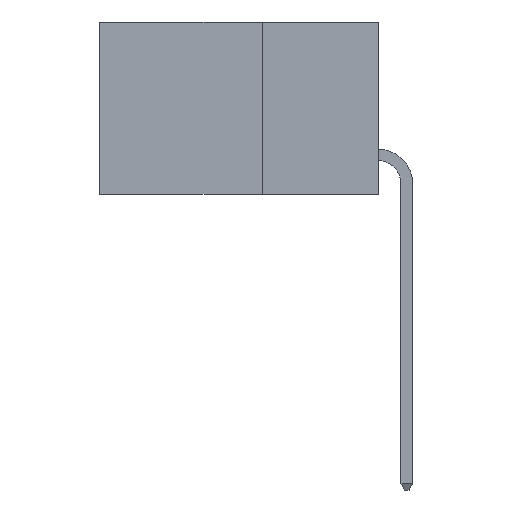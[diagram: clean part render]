
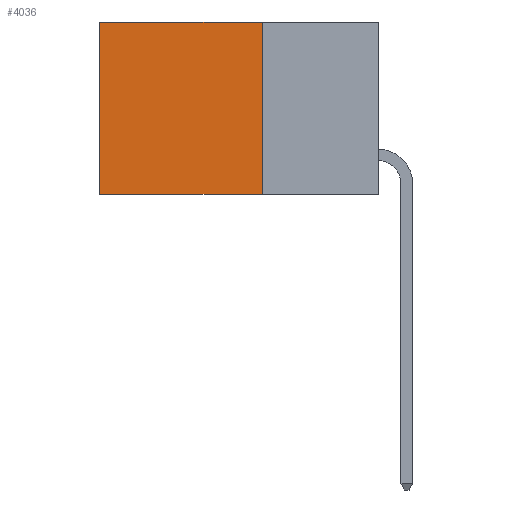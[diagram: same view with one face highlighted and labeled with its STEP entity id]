
A CAD part, left-side view. The second image highlights one B-rep face of the part: STEP entity #4036.
In plain terms, the highlighted planar face has unit normal (-1, 0, 0).
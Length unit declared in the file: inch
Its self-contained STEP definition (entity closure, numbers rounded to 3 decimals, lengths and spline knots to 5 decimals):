
#415 = VECTOR ( 'NONE', #8422, 39.37008 ) ;
#1345 = DIRECTION ( 'NONE',  ( 0., 0., -1. ) ) ;
#1356 = DIRECTION ( 'NONE',  ( 1., 0., 0. ) ) ;
#1359 = CARTESIAN_POINT ( 'NONE',  ( 0.2615, 0.25, -0.37 ) ) ;
#1370 = PLANE ( 'NONE',  #12226 ) ;
#1559 = CARTESIAN_POINT ( 'NONE',  ( 0.2615, 0.25, -0.37 ) ) ;
#1902 = DIRECTION ( 'NONE',  ( 0., 1., 0. ) ) ;
#2111 = EDGE_LOOP ( 'NONE', ( #6535, #9943, #9613, #9391 ) ) ;
#2649 = EDGE_CURVE ( 'NONE', #10400, #10882, #10931, .T. ) ;
#2899 = EDGE_CURVE ( 'NONE', #6331, #10882, #8090, .T. ) ;
#3427 = VECTOR ( 'NONE', #12170, 39.37008 ) ;
#3545 = CARTESIAN_POINT ( 'NONE',  ( 0.2615, 0.25, -0.37 ) ) ;
#4036 = ADVANCED_FACE ( 'NONE', ( #6282 ), #1370, .F. ) ;
#4127 = CARTESIAN_POINT ( 'NONE',  ( 0.2615, 0.6, -0.37 ) ) ;
#4901 = CARTESIAN_POINT ( 'NONE',  ( 0.2615, 0.25, 0. ) ) ;
#5163 = DIRECTION ( 'NONE',  ( 0., 1., 0. ) ) ;
#5191 = VECTOR ( 'NONE', #5163, 39.37008 ) ;
#6282 = FACE_OUTER_BOUND ( 'NONE', #2111, .T. ) ;
#6331 = VERTEX_POINT ( 'NONE', #10283 ) ;
#6388 = EDGE_CURVE ( 'NONE', #12286, #10400, #8079, .T. ) ;
#6535 = ORIENTED_EDGE ( 'NONE', *, *, #2899, .T. ) ;
#6746 = CARTESIAN_POINT ( 'NONE',  ( 0.2615, 0.25, -0.37 ) ) ;
#7443 = EDGE_CURVE ( 'NONE', #12286, #6331, #9744, .T. ) ;
#8079 = LINE ( 'NONE', #6746, #3427 ) ;
#8090 = LINE ( 'NONE', #8499, #415 ) ;
#8240 = VECTOR ( 'NONE', #1902, 39.37008 ) ;
#8422 = DIRECTION ( 'NONE',  ( 0., 0., -1. ) ) ;
#8499 = CARTESIAN_POINT ( 'NONE',  ( 0.2615, 0.6, -0.37 ) ) ;
#9391 = ORIENTED_EDGE ( 'NONE', *, *, #7443, .T. ) ;
#9613 = ORIENTED_EDGE ( 'NONE', *, *, #6388, .F. ) ;
#9744 = LINE ( 'NONE', #11536, #5191 ) ;
#9943 = ORIENTED_EDGE ( 'NONE', *, *, #2649, .F. ) ;
#10283 = CARTESIAN_POINT ( 'NONE',  ( 0.2615, 0.6, 0. ) ) ;
#10400 = VERTEX_POINT ( 'NONE', #1359 ) ;
#10882 = VERTEX_POINT ( 'NONE', #4127 ) ;
#10931 = LINE ( 'NONE', #3545, #8240 ) ;
#11536 = CARTESIAN_POINT ( 'NONE',  ( 0.2615, 0.25, 0. ) ) ;
#12170 = DIRECTION ( 'NONE',  ( 0., 0., -1. ) ) ;
#12226 = AXIS2_PLACEMENT_3D ( 'NONE', #1559, #1356, #1345 ) ;
#12286 = VERTEX_POINT ( 'NONE', #4901 ) ;
